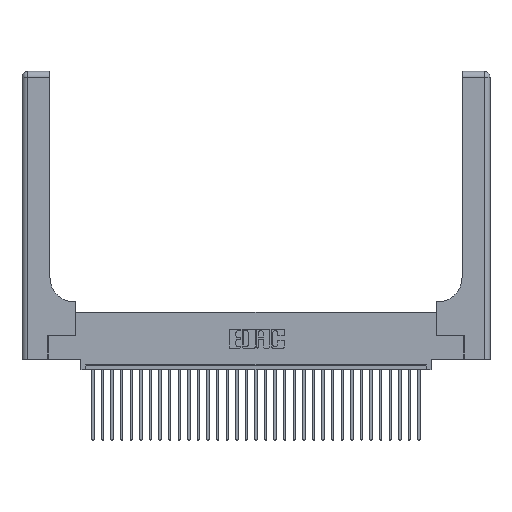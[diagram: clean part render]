
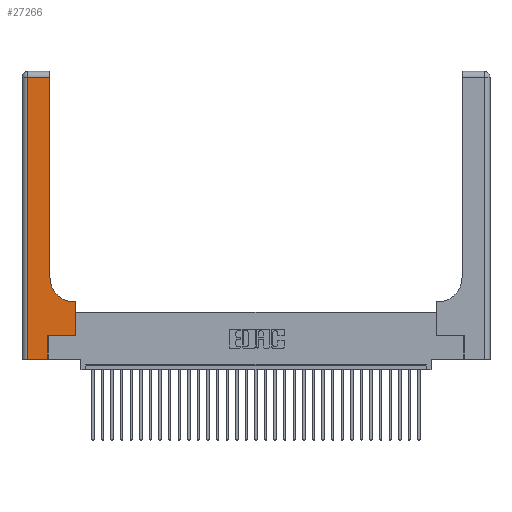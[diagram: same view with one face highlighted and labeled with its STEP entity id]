
A CAD part, top view. The second image highlights one B-rep face of the part: STEP entity #27266.
In plain terms, the highlighted planar face has unit normal (0, 0, 1).
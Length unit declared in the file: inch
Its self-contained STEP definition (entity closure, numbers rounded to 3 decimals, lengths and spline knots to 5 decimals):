
#209 = CARTESIAN_POINT ( 'NONE',  ( 0., 0., 0.37 ) ) ;
#300 = VECTOR ( 'NONE', #9681, 39.37008 ) ;
#514 = CARTESIAN_POINT ( 'NONE',  ( 0., 2.94, 0.37 ) ) ;
#529 = DIRECTION ( 'NONE',  ( 1., 0., 0. ) ) ;
#950 = LINE ( 'NONE', #7177, #15173 ) ;
#1099 = DIRECTION ( 'NONE',  ( 0., 0., -1. ) ) ;
#1282 = LINE ( 'NONE', #25203, #28082 ) ;
#1288 = ORIENTED_EDGE ( 'NONE', *, *, #19381, .T. ) ;
#1336 = CARTESIAN_POINT ( 'NONE',  ( 0.5415, 0.85, 0.37 ) ) ;
#1365 = VERTEX_POINT ( 'NONE', #18104 ) ;
#1818 = CARTESIAN_POINT ( 'NONE',  ( 0.2915, 2.94, 0.37 ) ) ;
#1968 = FACE_OUTER_BOUND ( 'NONE', #6698, .T. ) ;
#2239 = VECTOR ( 'NONE', #15530, 39.37008 ) ;
#2482 = CARTESIAN_POINT ( 'NONE',  ( 0.269, 0.25, 0.37 ) ) ;
#3851 = CARTESIAN_POINT ( 'NONE',  ( 0.2915, 0.6, 0.37 ) ) ;
#4205 = CARTESIAN_POINT ( 'NONE',  ( 0.5585, 0.25, 0.37 ) ) ;
#4791 = ORIENTED_EDGE ( 'NONE', *, *, #10710, .T. ) ;
#6013 = LINE ( 'NONE', #3851, #22163 ) ;
#6608 = CARTESIAN_POINT ( 'NONE',  ( 0.269, 0., 0.37 ) ) ;
#6698 = EDGE_LOOP ( 'NONE', ( #25200, #4791, #9271, #15032, #26770, #32245, #10692, #8089, #1288 ) ) ;
#7177 = CARTESIAN_POINT ( 'NONE',  ( 0.5585, 0.25, 0.37 ) ) ;
#7401 = PLANE ( 'NONE',  #30893 ) ;
#7420 = EDGE_CURVE ( 'NONE', #11016, #12472, #21282, .T. ) ;
#8089 = ORIENTED_EDGE ( 'NONE', *, *, #8719, .T. ) ;
#8719 = EDGE_CURVE ( 'NONE', #10343, #25676, #6013, .T. ) ;
#9254 = CARTESIAN_POINT ( 'NONE',  ( 0.2915, 3., 0.37 ) ) ;
#9271 = ORIENTED_EDGE ( 'NONE', *, *, #10332, .T. ) ;
#9290 = DIRECTION ( 'NONE',  ( -1., 0., 0. ) ) ;
#9423 = LINE ( 'NONE', #209, #29495 ) ;
#9681 = DIRECTION ( 'NONE',  ( 1., 0., 0. ) ) ;
#10142 = DIRECTION ( 'NONE',  ( 0., 1., 0. ) ) ;
#10332 = EDGE_CURVE ( 'NONE', #11747, #1365, #1282, .T. ) ;
#10343 = VERTEX_POINT ( 'NONE', #27837 ) ;
#10692 = ORIENTED_EDGE ( 'NONE', *, *, #11601, .T. ) ;
#10710 = EDGE_CURVE ( 'NONE', #22597, #11747, #23889, .T. ) ;
#11016 = VERTEX_POINT ( 'NONE', #21093 ) ;
#11601 = EDGE_CURVE ( 'NONE', #12472, #10343, #950, .T. ) ;
#11747 = VERTEX_POINT ( 'NONE', #20851 ) ;
#12165 = VERTEX_POINT ( 'NONE', #16232 ) ;
#12466 = DIRECTION ( 'NONE',  ( -1., 0., 0. ) ) ;
#12472 = VERTEX_POINT ( 'NONE', #4205 ) ;
#13154 = EDGE_CURVE ( 'NONE', #12165, #22597, #28118, .T. ) ;
#13324 = CARTESIAN_POINT ( 'NONE',  ( 0.269, 0., 0.37 ) ) ;
#14758 = VERTEX_POINT ( 'NONE', #6608 ) ;
#15032 = ORIENTED_EDGE ( 'NONE', *, *, #19799, .T. ) ;
#15173 = VECTOR ( 'NONE', #29513, 39.37008 ) ;
#15530 = DIRECTION ( 'NONE',  ( -1., 0., 0. ) ) ;
#16232 = CARTESIAN_POINT ( 'NONE',  ( 0.2915, 0.85, 0.37 ) ) ;
#18104 = CARTESIAN_POINT ( 'NONE',  ( 0.06, 0., 0.37 ) ) ;
#18664 = CARTESIAN_POINT ( 'NONE',  ( 0.5415, 0.6, 0.37 ) ) ;
#19381 = EDGE_CURVE ( 'NONE', #25676, #12165, #32260, .T. ) ;
#19799 = EDGE_CURVE ( 'NONE', #1365, #14758, #9423, .T. ) ;
#20670 = DIRECTION ( 'NONE',  ( 0., 1., 0. ) ) ;
#20851 = CARTESIAN_POINT ( 'NONE',  ( 0.06, 2.94, 0.37 ) ) ;
#21093 = CARTESIAN_POINT ( 'NONE',  ( 0.269, 0.25, 0.37 ) ) ;
#21282 = LINE ( 'NONE', #2482, #300 ) ;
#22163 = VECTOR ( 'NONE', #9290, 39.37008 ) ;
#22191 = VECTOR ( 'NONE', #10142, 39.37008 ) ;
#22597 = VERTEX_POINT ( 'NONE', #1818 ) ;
#23889 = LINE ( 'NONE', #514, #2239 ) ;
#24624 = AXIS2_PLACEMENT_3D ( 'NONE', #1336, #1099, #26338 ) ;
#25004 = CARTESIAN_POINT ( 'NONE',  ( 0., 3., 0.37 ) ) ;
#25200 = ORIENTED_EDGE ( 'NONE', *, *, #13154, .T. ) ;
#25203 = CARTESIAN_POINT ( 'NONE',  ( 0.06, 3., 0.37 ) ) ;
#25233 = DIRECTION ( 'NONE',  ( 0., -1., 0. ) ) ;
#25600 = EDGE_CURVE ( 'NONE', #14758, #11016, #27312, .T. ) ;
#25676 = VERTEX_POINT ( 'NONE', #18664 ) ;
#26338 = DIRECTION ( 'NONE',  ( 1., 0., 0. ) ) ;
#26493 = VECTOR ( 'NONE', #20670, 39.37008 ) ;
#26770 = ORIENTED_EDGE ( 'NONE', *, *, #25600, .T. ) ;
#27266 = ADVANCED_FACE ( 'NONE', ( #1968 ), #7401, .F. ) ;
#27312 = LINE ( 'NONE', #13324, #26493 ) ;
#27535 = DIRECTION ( 'NONE',  ( 0., 0., -1. ) ) ;
#27837 = CARTESIAN_POINT ( 'NONE',  ( 0.5585, 0.6, 0.37 ) ) ;
#28082 = VECTOR ( 'NONE', #25233, 39.37008 ) ;
#28118 = LINE ( 'NONE', #9254, #22191 ) ;
#29495 = VECTOR ( 'NONE', #529, 39.37008 ) ;
#29513 = DIRECTION ( 'NONE',  ( 0., 1., 0. ) ) ;
#30893 = AXIS2_PLACEMENT_3D ( 'NONE', #25004, #27535, #12466 ) ;
#32245 = ORIENTED_EDGE ( 'NONE', *, *, #7420, .T. ) ;
#32260 = CIRCLE ( 'NONE', #24624, 0.25 ) ;
